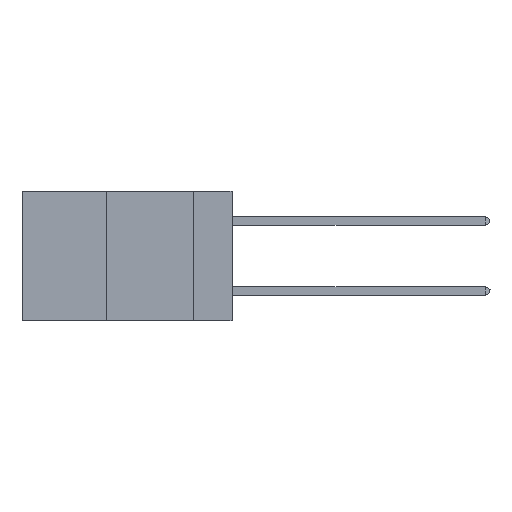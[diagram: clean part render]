
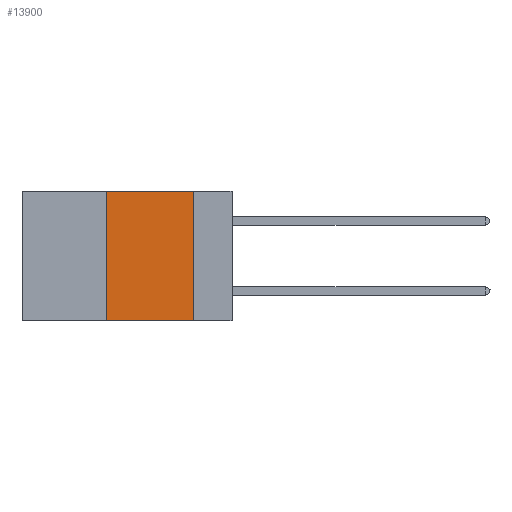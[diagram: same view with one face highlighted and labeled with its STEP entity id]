
A CAD part, left-side view. The second image highlights one B-rep face of the part: STEP entity #13900.
In plain terms, the highlighted planar face has unit normal (-1, 0, 0).
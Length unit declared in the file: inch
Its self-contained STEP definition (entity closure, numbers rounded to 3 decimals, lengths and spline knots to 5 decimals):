
#845 = ORIENTED_EDGE ( 'NONE', *, *, #18682, .F. ) ;
#1479 = DIRECTION ( 'NONE',  ( 0., 0., -1. ) ) ;
#2674 = DIRECTION ( 'NONE',  ( 0., -1., 0. ) ) ;
#2710 = VECTOR ( 'NONE', #2674, 39.37008 ) ;
#2775 = CARTESIAN_POINT ( 'NONE',  ( 0., 0.11, -0.37 ) ) ;
#3882 = CARTESIAN_POINT ( 'NONE',  ( 0., 0.36, 0. ) ) ;
#3987 = CARTESIAN_POINT ( 'NONE',  ( 0., 0.36, 0. ) ) ;
#4076 = ORIENTED_EDGE ( 'NONE', *, *, #8213, .T. ) ;
#4241 = LINE ( 'NONE', #16726, #2710 ) ;
#7501 = PLANE ( 'NONE',  #23518 ) ;
#8213 = EDGE_CURVE ( 'NONE', #11534, #10152, #4241, .T. ) ;
#8600 = EDGE_CURVE ( 'NONE', #11534, #14597, #20945, .T. ) ;
#9141 = CARTESIAN_POINT ( 'NONE',  ( 0., 0.11, 0. ) ) ;
#9896 = DIRECTION ( 'NONE',  ( 0., -1., 0. ) ) ;
#10152 = VERTEX_POINT ( 'NONE', #2775 ) ;
#10704 = LINE ( 'NONE', #9141, #13210 ) ;
#10934 = VERTEX_POINT ( 'NONE', #15874 ) ;
#11534 = VERTEX_POINT ( 'NONE', #11957 ) ;
#11744 = ORIENTED_EDGE ( 'NONE', *, *, #8600, .F. ) ;
#11957 = CARTESIAN_POINT ( 'NONE',  ( 0., 0.36, -0.37 ) ) ;
#13210 = VECTOR ( 'NONE', #1479, 39.37008 ) ;
#13506 = ORIENTED_EDGE ( 'NONE', *, *, #22940, .F. ) ;
#13900 = ADVANCED_FACE ( 'NONE', ( #19281 ), #7501, .F. ) ;
#14597 = VERTEX_POINT ( 'NONE', #3987 ) ;
#15226 = DIRECTION ( 'NONE',  ( 1., 0., 0. ) ) ;
#15835 = VECTOR ( 'NONE', #9896, 39.37008 ) ;
#15874 = CARTESIAN_POINT ( 'NONE',  ( 0., 0.11, 0. ) ) ;
#16726 = CARTESIAN_POINT ( 'NONE',  ( 0., 0.6, -0.37 ) ) ;
#17932 = DIRECTION ( 'NONE',  ( 0., 0., 1. ) ) ;
#18682 = EDGE_CURVE ( 'NONE', #14597, #10934, #21081, .T. ) ;
#19281 = FACE_OUTER_BOUND ( 'NONE', #23557, .T. ) ;
#20945 = LINE ( 'NONE', #3882, #23716 ) ;
#21081 = LINE ( 'NONE', #21627, #15835 ) ;
#21344 = DIRECTION ( 'NONE',  ( 0., 0., -1. ) ) ;
#21627 = CARTESIAN_POINT ( 'NONE',  ( 0., 0.6, 0. ) ) ;
#22940 = EDGE_CURVE ( 'NONE', #10934, #10152, #10704, .T. ) ;
#23518 = AXIS2_PLACEMENT_3D ( 'NONE', #25396, #15226, #21344 ) ;
#23557 = EDGE_LOOP ( 'NONE', ( #13506, #845, #11744, #4076 ) ) ;
#23716 = VECTOR ( 'NONE', #17932, 39.37008 ) ;
#25396 = CARTESIAN_POINT ( 'NONE',  ( 0., 0.6, 0. ) ) ;
